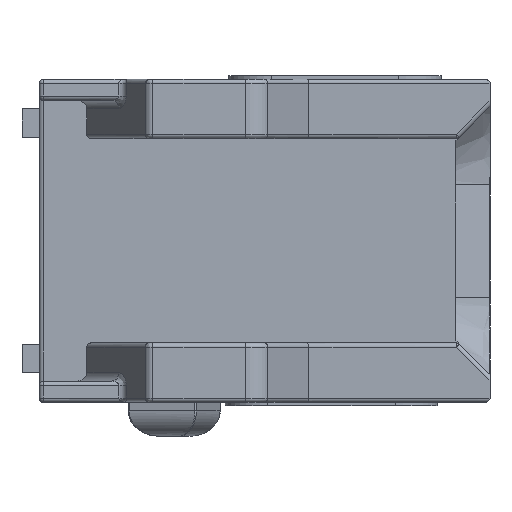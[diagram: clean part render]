
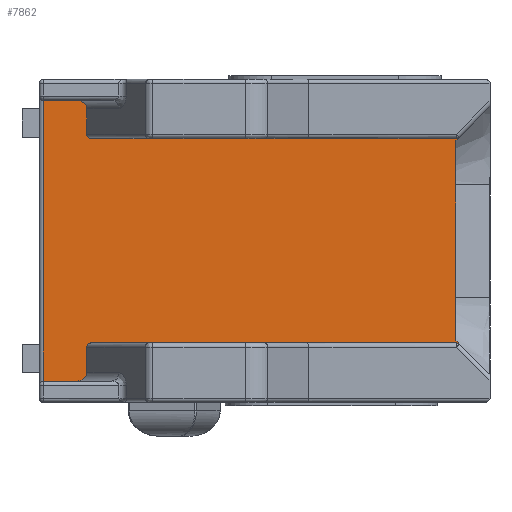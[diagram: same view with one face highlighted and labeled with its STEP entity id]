
A CAD part, left-side view. The second image highlights one B-rep face of the part: STEP entity #7862.
In plain terms, the highlighted planar face has unit normal (-1, 0, 0).
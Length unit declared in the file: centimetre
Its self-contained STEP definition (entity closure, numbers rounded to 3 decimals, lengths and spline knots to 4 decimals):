
#393=PLANE($,#8489);
#760=LINE($,#12957,#1437);
#764=LINE($,#13034,#1441);
#804=LINE($,#13355,#1481);
#879=LINE($,#14190,#1556);
#884=LINE($,#14328,#1561);
#885=LINE($,#14330,#1562);
#886=LINE($,#14333,#1563);
#887=LINE($,#14335,#1564);
#888=LINE($,#14336,#1565);
#889=LINE($,#14338,#1566);
#1437=VECTOR($,#9470,0.3963);
#1441=VECTOR($,#9494,0.3963);
#1481=VECTOR($,#9702,3.3);
#1556=VECTOR($,#9911,0.056);
#1561=VECTOR($,#9936,0.3);
#1562=VECTOR($,#9937,0.3);
#1563=VECTOR($,#9940,4.2848);
#1564=VECTOR($,#9941,2.35);
#1565=VECTOR($,#9942,0.0561);
#1566=VECTOR($,#9943,4.2848);
#2236=FACE_OUTER_BOUND($,#2711,.T.);
#2711=EDGE_LOOP($,(#6400,#6401,#6402,#6403,#6404,#6405,#6406,#6407,#6408,
#6409,#6410,#6411,#6412,#6413,#6414,#6415));
#2960=ELLIPSE($,#8320,0.1155,0.1);
#2969=ELLIPSE($,#8343,0.1155,0.1);
#2983=ELLIPSE($,#8490,0.0577,0.05);
#2984=ELLIPSE($,#8491,0.0577,0.05);
#3144=CIRCLE($,#8478,0.05);
#3148=CIRCLE($,#8486,0.05);
#3393=VERTEX_POINT($,#11694);
#3529=VERTEX_POINT($,#12955);
#3530=VERTEX_POINT($,#12959);
#3535=VERTEX_POINT($,#13030);
#3537=VERTEX_POINT($,#13033);
#3546=VERTEX_POINT($,#13093);
#3657=VERTEX_POINT($,#14181);
#3658=VERTEX_POINT($,#14183);
#3659=VERTEX_POINT($,#14187);
#3660=VERTEX_POINT($,#14189);
#3663=VERTEX_POINT($,#14201);
#3665=VERTEX_POINT($,#14327);
#3666=VERTEX_POINT($,#14329);
#3667=VERTEX_POINT($,#14331);
#3668=VERTEX_POINT($,#14334);
#3669=VERTEX_POINT($,#14337);
#4414=EDGE_CURVE($,#3393,#3529,#760,.T.);
#4415=EDGE_CURVE($,#3530,#3529,#2960,.T.);
#4425=EDGE_CURVE($,#3535,#3537,#764,.T.);
#4441=EDGE_CURVE($,#3535,#3546,#2969,.T.);
#4516=EDGE_CURVE($,#3537,#3393,#804,.T.);
#4649=EDGE_CURVE($,#3657,#3658,#3144,.F.);
#4652=EDGE_CURVE($,#3659,#3660,#879,.T.);
#4658=EDGE_CURVE($,#3660,#3663,#3148,.F.);
#4663=EDGE_CURVE($,#3665,#3530,#884,.T.);
#4664=EDGE_CURVE($,#3546,#3666,#885,.T.);
#4665=EDGE_CURVE($,#3667,#3666,#2983,.F.);
#4666=EDGE_CURVE($,#3663,#3667,#886,.T.);
#4667=EDGE_CURVE($,#3659,#3668,#887,.F.);
#4668=EDGE_CURVE($,#3658,#3668,#888,.T.);
#4669=EDGE_CURVE($,#3669,#3657,#889,.T.);
#4670=EDGE_CURVE($,#3665,#3669,#2984,.F.);
#6400=ORIENTED_EDGE($,*,*,#4663,.T.);
#6401=ORIENTED_EDGE($,*,*,#4415,.T.);
#6402=ORIENTED_EDGE($,*,*,#4414,.F.);
#6403=ORIENTED_EDGE($,*,*,#4516,.F.);
#6404=ORIENTED_EDGE($,*,*,#4425,.F.);
#6405=ORIENTED_EDGE($,*,*,#4441,.T.);
#6406=ORIENTED_EDGE($,*,*,#4664,.T.);
#6407=ORIENTED_EDGE($,*,*,#4665,.F.);
#6408=ORIENTED_EDGE($,*,*,#4666,.F.);
#6409=ORIENTED_EDGE($,*,*,#4658,.F.);
#6410=ORIENTED_EDGE($,*,*,#4652,.F.);
#6411=ORIENTED_EDGE($,*,*,#4667,.T.);
#6412=ORIENTED_EDGE($,*,*,#4668,.F.);
#6413=ORIENTED_EDGE($,*,*,#4649,.F.);
#6414=ORIENTED_EDGE($,*,*,#4669,.F.);
#6415=ORIENTED_EDGE($,*,*,#4670,.F.);
#7862=ADVANCED_FACE($,(#2236),#393,.F.);
#8320=AXIS2_PLACEMENT_3D($,#12960,#9473,#9474);
#8343=AXIS2_PLACEMENT_3D($,#13094,#9529,#9530);
#8478=AXIS2_PLACEMENT_3D($,#14184,#9905,#9906);
#8486=AXIS2_PLACEMENT_3D($,#14202,#9926,#9927);
#8489=AXIS2_PLACEMENT_3D($,#14326,#9934,#9935);
#8490=AXIS2_PLACEMENT_3D($,#14332,#9938,#9939);
#8491=AXIS2_PLACEMENT_3D($,#14339,#9944,#9945);
#9470=DIRECTION($,(0.,-1.,0.));
#9473=DIRECTION('center_axis',(-1.,0.,0.));
#9474=DIRECTION('ref_axis',(0.,-1.,0.));
#9494=DIRECTION($,(0.,1.,0.));
#9529=DIRECTION('center_axis',(-1.,0.,0.));
#9530=DIRECTION('ref_axis',(0.,-1.,0.));
#9702=DIRECTION($,(0.,0.,1.));
#9905=DIRECTION('center_axis',(1.,0.,0.));
#9906=DIRECTION('ref_axis',(0.,-0.383,-0.924));
#9911=DIRECTION($,(0.,-0.707,-0.707));
#9926=DIRECTION('center_axis',(1.,0.,0.));
#9927=DIRECTION('ref_axis',(0.,-0.383,0.924));
#9934=DIRECTION('center_axis',(1.,0.,0.));
#9935=DIRECTION('ref_axis',(0.,0.,-1.));
#9936=DIRECTION($,(0.,0.,1.));
#9937=DIRECTION($,(0.,0.,1.));
#9938=DIRECTION('center_axis',(1.,0.,0.));
#9939=DIRECTION('ref_axis',(0.,1.,0.));
#9940=DIRECTION($,(0.,1.,0.));
#9941=DIRECTION($,(0.,0.,-1.));
#9942=DIRECTION($,(0.,0.707,-0.707));
#9943=DIRECTION($,(0.,-1.,0.));
#9944=DIRECTION('center_axis',(1.,0.,0.));
#9945=DIRECTION('ref_axis',(0.,1.,0.));
#11694=CARTESIAN_POINT('',(-8.24,-10.879,1.75));
#12955=CARTESIAN_POINT('',(-8.24,-11.2753,1.75));
#12957=CARTESIAN_POINT($,(-8.24,-13.284,1.75));
#12959=CARTESIAN_POINT('',(-8.24,-11.3907,1.65));
#12960=CARTESIAN_POINT('Origin',(-8.24,-11.2753,1.65));
#13030=CARTESIAN_POINT('',(-8.24,-11.2753,-1.55));
#13033=CARTESIAN_POINT('',(-8.24,-10.879,-1.55));
#13034=CARTESIAN_POINT($,(-8.24,-13.1547,-1.55));
#13093=CARTESIAN_POINT('',(-8.24,-11.3907,-1.45));
#13094=CARTESIAN_POINT('Origin',(-8.24,-11.2753,-1.45));
#13355=CARTESIAN_POINT($,(-8.24,-10.879,0.1));
#14181=CARTESIAN_POINT('',(-8.24,-15.7333,1.3));
#14183=CARTESIAN_POINT('',(-8.24,-15.7686,1.3146));
#14184=CARTESIAN_POINT('Origin',(-8.24,-15.7333,1.35));
#14187=CARTESIAN_POINT('',(-8.24,-15.729,-1.075));
#14189=CARTESIAN_POINT('',(-8.24,-15.7686,-1.1146));
#14190=CARTESIAN_POINT($,(-8.24,-14.8815,-0.2275));
#14201=CARTESIAN_POINT('',(-8.24,-15.7332,-1.1));
#14202=CARTESIAN_POINT('Origin',(-8.24,-15.7332,-1.15));
#14326=CARTESIAN_POINT('Origin',(-8.24,-13.1141,0.1));
#14327=CARTESIAN_POINT('',(-8.24,-11.3907,1.35));
#14328=CARTESIAN_POINT($,(-8.24,-11.3907,-0.91));
#14329=CARTESIAN_POINT('',(-8.24,-11.3907,-1.15));
#14330=CARTESIAN_POINT($,(-8.24,-11.3907,-0.91));
#14331=CARTESIAN_POINT('',(-8.24,-11.4485,-1.1));
#14332=CARTESIAN_POINT('Origin',(-8.24,-11.4485,-1.15));
#14333=CARTESIAN_POINT($,(-8.24,-13.1547,-1.1));
#14334=CARTESIAN_POINT('',(-8.24,-15.729,1.275));
#14335=CARTESIAN_POINT($,(-8.24,-15.729,0.917));
#14336=CARTESIAN_POINT($,(-8.24,-14.8815,0.4275));
#14337=CARTESIAN_POINT('',(-8.24,-11.4485,1.3));
#14338=CARTESIAN_POINT($,(-8.24,-13.284,1.3));
#14339=CARTESIAN_POINT('Origin',(-8.24,-11.4485,1.35));
